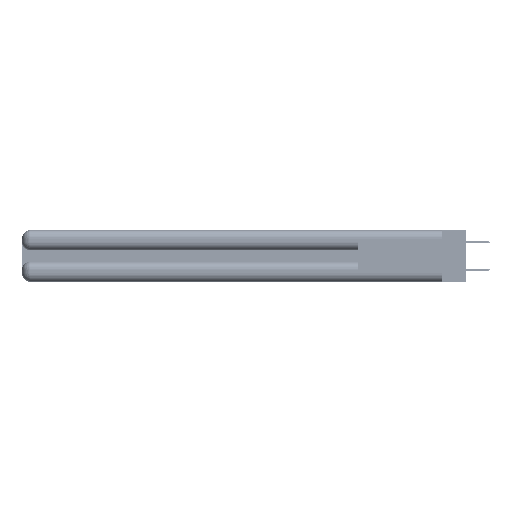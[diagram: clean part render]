
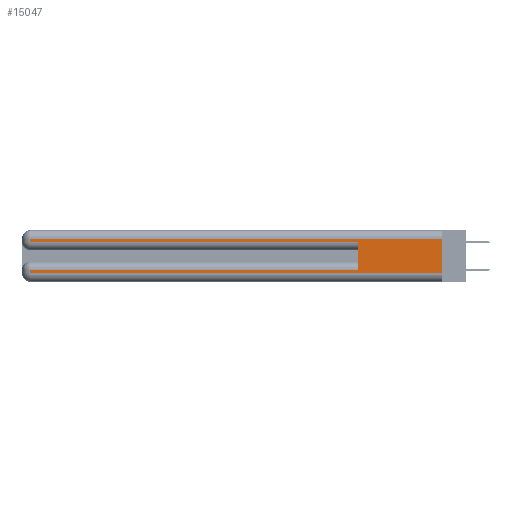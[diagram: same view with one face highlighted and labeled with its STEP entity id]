
A CAD part, left-side view. The second image highlights one B-rep face of the part: STEP entity #15047.
In plain terms, the highlighted planar face has unit normal (-1, 0, 0).
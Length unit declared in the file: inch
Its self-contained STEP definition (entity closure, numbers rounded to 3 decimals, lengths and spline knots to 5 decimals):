
#24 = VERTEX_POINT ( 'NONE', #4310 ) ;
#1073 = VECTOR ( 'NONE', #35545, 39.37008 ) ;
#1577 = CARTESIAN_POINT ( 'NONE',  ( 0., 2.94, 0.37 ) ) ;
#2469 = CARTESIAN_POINT ( 'NONE',  ( 0., 0., 0.37 ) ) ;
#2640 = ORIENTED_EDGE ( 'NONE', *, *, #14350, .T. ) ;
#2971 = LINE ( 'NONE', #19454, #21386 ) ;
#3175 = LINE ( 'NONE', #10758, #46734 ) ;
#3710 = LINE ( 'NONE', #18577, #1073 ) ;
#4310 = CARTESIAN_POINT ( 'NONE',  ( 0., 0., 0.06 ) ) ;
#5012 = ORIENTED_EDGE ( 'NONE', *, *, #12674, .F. ) ;
#5089 = DIRECTION ( 'NONE',  ( 0., 0., -1. ) ) ;
#6807 = CARTESIAN_POINT ( 'NONE',  ( 0., 2.94, 0.285 ) ) ;
#7195 = ORIENTED_EDGE ( 'NONE', *, *, #50195, .T. ) ;
#8796 = LINE ( 'NONE', #37801, #32498 ) ;
#9591 = VERTEX_POINT ( 'NONE', #29486 ) ;
#9600 = VECTOR ( 'NONE', #31788, 39.37008 ) ;
#10369 = ORIENTED_EDGE ( 'NONE', *, *, #54449, .T. ) ;
#10758 = CARTESIAN_POINT ( 'NONE',  ( 0., 0.6, 0.145 ) ) ;
#11497 = PLANE ( 'NONE',  #29581 ) ;
#12674 = EDGE_CURVE ( 'NONE', #43612, #21516, #3175, .T. ) ;
#13659 = ORIENTED_EDGE ( 'NONE', *, *, #20284, .T. ) ;
#14350 = EDGE_CURVE ( 'NONE', #9591, #49162, #2971, .T. ) ;
#14480 = ORIENTED_EDGE ( 'NONE', *, *, #34472, .F. ) ;
#15047 = ADVANCED_FACE ( 'NONE', ( #51098 ), #11497, .F. ) ;
#17510 = DIRECTION ( 'NONE',  ( 0., -1., 0. ) ) ;
#18577 = CARTESIAN_POINT ( 'NONE',  ( 0., 0., 0.085 ) ) ;
#19454 = CARTESIAN_POINT ( 'NONE',  ( 0., 2.94, 0.37 ) ) ;
#20284 = EDGE_CURVE ( 'NONE', #43612, #32354, #3710, .T. ) ;
#21386 = VECTOR ( 'NONE', #44596, 39.37008 ) ;
#21516 = VERTEX_POINT ( 'NONE', #22119 ) ;
#21700 = CARTESIAN_POINT ( 'NONE',  ( 0., 2.94, 0.085 ) ) ;
#22119 = CARTESIAN_POINT ( 'NONE',  ( 0., 0.6, 0.285 ) ) ;
#22532 = CARTESIAN_POINT ( 'NONE',  ( 0., 0., 0.31 ) ) ;
#23069 = CARTESIAN_POINT ( 'NONE',  ( 0., 0., 0.37 ) ) ;
#23556 = VECTOR ( 'NONE', #48382, 39.37008 ) ;
#24083 = LINE ( 'NONE', #35700, #9600 ) ;
#27151 = CARTESIAN_POINT ( 'NONE',  ( 0., 0., 0.31 ) ) ;
#27837 = EDGE_CURVE ( 'NONE', #32354, #34191, #52238, .T. ) ;
#29486 = CARTESIAN_POINT ( 'NONE',  ( 0., 2.94, 0.31 ) ) ;
#29581 = AXIS2_PLACEMENT_3D ( 'NONE', #2469, #41001, #36191 ) ;
#30598 = CARTESIAN_POINT ( 'NONE',  ( 0., 0.6, 0.085 ) ) ;
#31788 = DIRECTION ( 'NONE',  ( 0., -1., 0. ) ) ;
#32354 = VERTEX_POINT ( 'NONE', #21700 ) ;
#32498 = VECTOR ( 'NONE', #17510, 39.37008 ) ;
#33412 = ORIENTED_EDGE ( 'NONE', *, *, #35820, .T. ) ;
#34191 = VERTEX_POINT ( 'NONE', #46928 ) ;
#34472 = EDGE_CURVE ( 'NONE', #44935, #24, #41429, .T. ) ;
#35545 = DIRECTION ( 'NONE',  ( 0., 1., 0. ) ) ;
#35700 = CARTESIAN_POINT ( 'NONE',  ( 0., 0., 0.06 ) ) ;
#35820 = EDGE_CURVE ( 'NONE', #34191, #24, #24083, .T. ) ;
#36191 = DIRECTION ( 'NONE',  ( 0., 0., -1. ) ) ;
#37801 = CARTESIAN_POINT ( 'NONE',  ( 0., 0., 0.285 ) ) ;
#41001 = DIRECTION ( 'NONE',  ( 1., 0., 0. ) ) ;
#41429 = LINE ( 'NONE', #23069, #23556 ) ;
#42171 = VECTOR ( 'NONE', #52317, 39.37008 ) ;
#43612 = VERTEX_POINT ( 'NONE', #30598 ) ;
#43648 = VECTOR ( 'NONE', #5089, 39.37008 ) ;
#44596 = DIRECTION ( 'NONE',  ( 0., 0., -1. ) ) ;
#44935 = VERTEX_POINT ( 'NONE', #22532 ) ;
#45311 = ORIENTED_EDGE ( 'NONE', *, *, #27837, .T. ) ;
#46034 = EDGE_LOOP ( 'NONE', ( #14480, #10369, #2640, #7195, #5012, #13659, #45311, #33412 ) ) ;
#46734 = VECTOR ( 'NONE', #49219, 39.37008 ) ;
#46928 = CARTESIAN_POINT ( 'NONE',  ( 0., 2.94, 0.06 ) ) ;
#48382 = DIRECTION ( 'NONE',  ( 0., 0., -1. ) ) ;
#48793 = LINE ( 'NONE', #27151, #42171 ) ;
#49162 = VERTEX_POINT ( 'NONE', #6807 ) ;
#49219 = DIRECTION ( 'NONE',  ( 0., 0., 1. ) ) ;
#50195 = EDGE_CURVE ( 'NONE', #49162, #21516, #8796, .T. ) ;
#51098 = FACE_OUTER_BOUND ( 'NONE', #46034, .T. ) ;
#52238 = LINE ( 'NONE', #1577, #43648 ) ;
#52317 = DIRECTION ( 'NONE',  ( 0., 1., 0. ) ) ;
#54449 = EDGE_CURVE ( 'NONE', #44935, #9591, #48793, .T. ) ;
